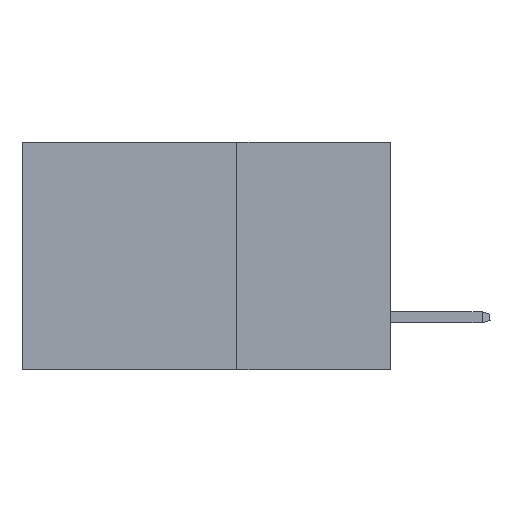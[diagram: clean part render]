
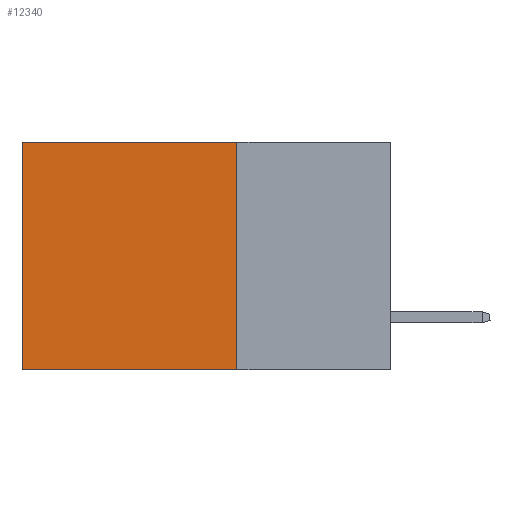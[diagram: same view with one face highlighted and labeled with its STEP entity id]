
A CAD part, left-side view. The second image highlights one B-rep face of the part: STEP entity #12340.
In plain terms, the highlighted planar face has unit normal (-1, 0, 0).
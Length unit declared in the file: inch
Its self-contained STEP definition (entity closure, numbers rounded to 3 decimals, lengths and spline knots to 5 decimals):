
#125 = VERTEX_POINT ( 'NONE', #2049 ) ;
#1395 = CARTESIAN_POINT ( 'NONE',  ( 0.2875, 0.25, 0. ) ) ;
#1658 = PLANE ( 'NONE',  #3129 ) ;
#2049 = CARTESIAN_POINT ( 'NONE',  ( 0.2875, 0.6, -0.37 ) ) ;
#3129 = AXIS2_PLACEMENT_3D ( 'NONE', #9616, #15872, #24237 ) ;
#3527 = LINE ( 'NONE', #8584, #20369 ) ;
#3974 = LINE ( 'NONE', #5616, #25960 ) ;
#4345 = EDGE_CURVE ( 'NONE', #22633, #17346, #14103, .T. ) ;
#5616 = CARTESIAN_POINT ( 'NONE',  ( 0.2875, 0.6, 0. ) ) ;
#5814 = ORIENTED_EDGE ( 'NONE', *, *, #4345, .T. ) ;
#6254 = EDGE_LOOP ( 'NONE', ( #6402, #12688, #11160, #5814 ) ) ;
#6402 = ORIENTED_EDGE ( 'NONE', *, *, #23153, .T. ) ;
#8584 = CARTESIAN_POINT ( 'NONE',  ( 0.2875, 0.25, -0.37 ) ) ;
#8921 = DIRECTION ( 'NONE',  ( 0., 0., -1. ) ) ;
#9236 = CARTESIAN_POINT ( 'NONE',  ( 0.2875, 0.25, -0.37 ) ) ;
#9616 = CARTESIAN_POINT ( 'NONE',  ( 0.2875, 0.25, 0. ) ) ;
#11160 = ORIENTED_EDGE ( 'NONE', *, *, #17284, .F. ) ;
#12340 = ADVANCED_FACE ( 'NONE', ( #23000 ), #1658, .F. ) ;
#12688 = ORIENTED_EDGE ( 'NONE', *, *, #20323, .F. ) ;
#13741 = DIRECTION ( 'NONE',  ( 0., 0., -1. ) ) ;
#14103 = LINE ( 'NONE', #25071, #20895 ) ;
#15332 = LINE ( 'NONE', #18191, #18592 ) ;
#15872 = DIRECTION ( 'NONE',  ( 1., 0., 0. ) ) ;
#16652 = DIRECTION ( 'NONE',  ( 0., 1., 0. ) ) ;
#17284 = EDGE_CURVE ( 'NONE', #22633, #25064, #15332, .T. ) ;
#17346 = VERTEX_POINT ( 'NONE', #25675 ) ;
#18191 = CARTESIAN_POINT ( 'NONE',  ( 0.2875, 0.25, 0. ) ) ;
#18592 = VECTOR ( 'NONE', #13741, 39.37008 ) ;
#18899 = DIRECTION ( 'NONE',  ( 0., 1., 0. ) ) ;
#20323 = EDGE_CURVE ( 'NONE', #25064, #125, #3527, .T. ) ;
#20369 = VECTOR ( 'NONE', #16652, 39.37008 ) ;
#20895 = VECTOR ( 'NONE', #18899, 39.37008 ) ;
#22633 = VERTEX_POINT ( 'NONE', #1395 ) ;
#23000 = FACE_OUTER_BOUND ( 'NONE', #6254, .T. ) ;
#23153 = EDGE_CURVE ( 'NONE', #17346, #125, #3974, .T. ) ;
#24237 = DIRECTION ( 'NONE',  ( 0., 0., -1. ) ) ;
#25064 = VERTEX_POINT ( 'NONE', #9236 ) ;
#25071 = CARTESIAN_POINT ( 'NONE',  ( 0.2875, 0.25, 0. ) ) ;
#25675 = CARTESIAN_POINT ( 'NONE',  ( 0.2875, 0.6, 0. ) ) ;
#25960 = VECTOR ( 'NONE', #8921, 39.37008 ) ;
